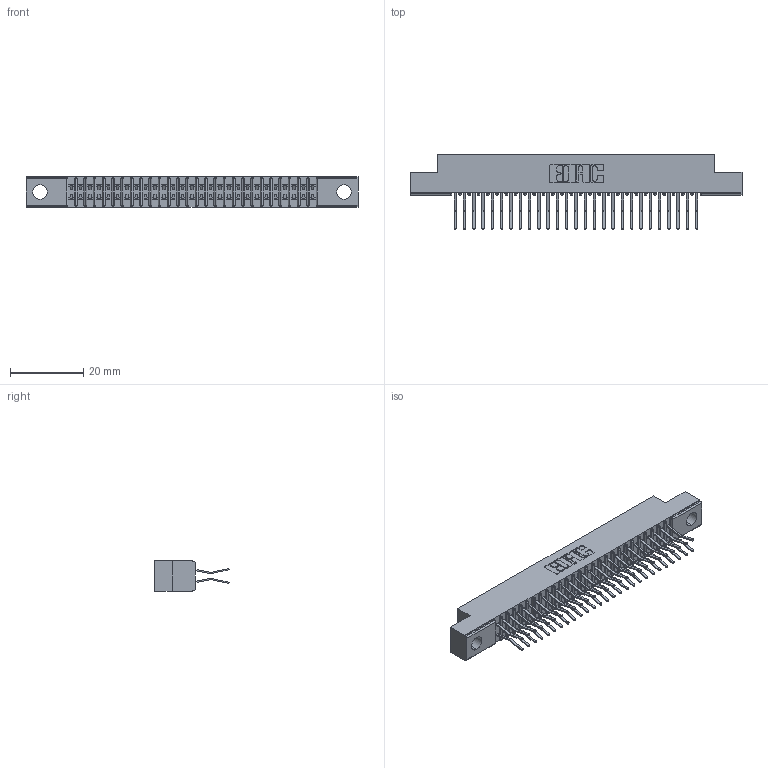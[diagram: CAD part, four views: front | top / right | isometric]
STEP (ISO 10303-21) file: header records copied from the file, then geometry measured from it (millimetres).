
FILE_DESCRIPTION (( 'STEP AP203' ), '1' );
FILE_NAME ('391-054-560-204.STEP', '2018-08-09T07:27:08', ( '' ), ( '' ), 'SwSTEP 2.0', 'SolidWorks 2016', '' );
FILE_SCHEMA (( 'CONFIG_CONTROL_DESIGN' ));
Length unit declared in the file: inch
Products named in the file (3): 341 Part_.156 (3.96) Dia Mounting Holes; 341-292-001_341-292-160; 391-054-560-204
Assembly tree (55 placements, depth 2):
  391-054-560-204
    341 Part_.156 (3.96) Dia Mounting Holes
    341-292-001_341-292-160  x54
Bounding box: 90.81 x 20.37 x 8.38 mm (x, y, z)
Volume: 5103.7 mm3; surface area: 11239.7 mm2
Topology: 55 solids, 55 shells, 3910 faces, 11341 edges, 7358 vertices
Faces by surface type: plane 2242, cylinder 1560, sphere 56, torus 52
Entity records: 35232 total; most frequent: CARTESIAN_POINT 5863, ORIENTED_EDGE 5822, DIRECTION 5697, EDGE_CURVE 2911, VECTOR 2337, LINE 2337, VERTEX_POINT 1846, AXIS2_PLACEMENT_3D 1680
